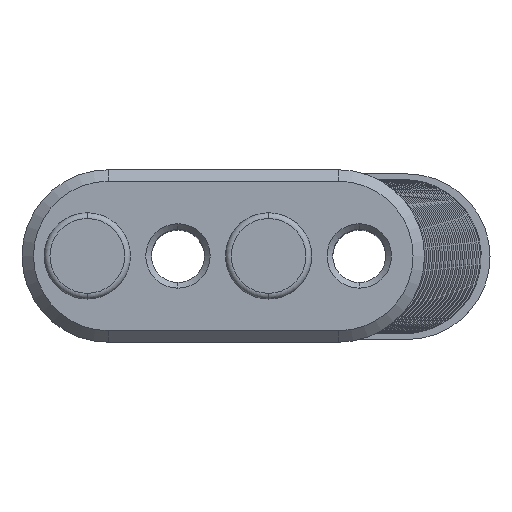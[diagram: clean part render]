
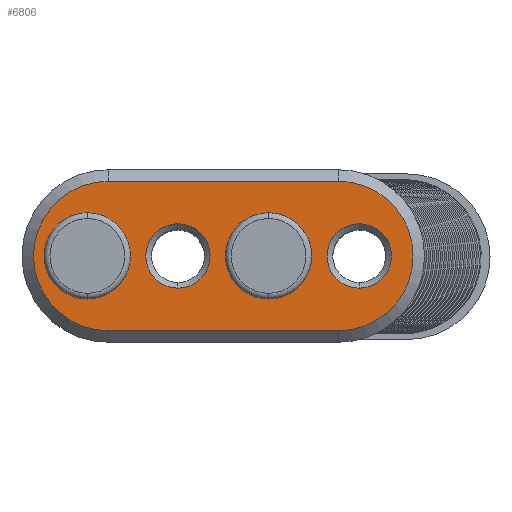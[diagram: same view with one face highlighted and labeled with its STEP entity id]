
A CAD part, top view. The second image highlights one B-rep face of the part: STEP entity #6806.
In plain terms, the highlighted planar face has unit normal (0, 0, 1).
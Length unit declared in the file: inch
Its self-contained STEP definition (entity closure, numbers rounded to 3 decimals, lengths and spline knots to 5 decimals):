
#20 = DIRECTION ( 'NONE',  ( 0., -1., 0. ) ) ;
#46 = EDGE_LOOP ( 'NONE', ( #3808, #5809 ) ) ;
#148 = FACE_BOUND ( 'NONE', #1703, .T. ) ;
#157 = AXIS2_PLACEMENT_3D ( 'NONE', #5842, #2017, #6483 ) ;
#225 = VERTEX_POINT ( 'NONE', #5051 ) ;
#270 = AXIS2_PLACEMENT_3D ( 'NONE', #5816, #649, #20 ) ;
#327 = DIRECTION ( 'NONE',  ( 0., 0., 1. ) ) ;
#331 = ORIENTED_EDGE ( 'NONE', *, *, #1484, .F. ) ;
#338 = DIRECTION ( 'NONE',  ( 0., 0., 1. ) ) ;
#632 = DIRECTION ( 'NONE',  ( 0., -1., 0. ) ) ;
#649 = DIRECTION ( 'NONE',  ( 0., 0., -1. ) ) ;
#738 = PLANE ( 'NONE',  #6042 ) ;
#747 = CARTESIAN_POINT ( 'NONE',  ( -0.5, -1.225, 1. ) ) ;
#770 = FACE_OUTER_BOUND ( 'NONE', #7071, .T. ) ;
#887 = VERTEX_POINT ( 'NONE', #1747 ) ;
#903 = DIRECTION ( 'NONE',  ( 0., 0., 1. ) ) ;
#988 = EDGE_CURVE ( 'NONE', #4217, #1450, #1202, .T. ) ;
#1107 = EDGE_CURVE ( 'NONE', #1518, #225, #6500, .T. ) ;
#1168 = AXIS2_PLACEMENT_3D ( 'NONE', #3433, #903, #4779 ) ;
#1202 = LINE ( 'NONE', #2324, #2707 ) ;
#1206 = EDGE_CURVE ( 'NONE', #1450, #887, #2096, .T. ) ;
#1263 = LINE ( 'NONE', #5788, #3372 ) ;
#1450 = VERTEX_POINT ( 'NONE', #3604 ) ;
#1484 = EDGE_CURVE ( 'NONE', #3655, #8273, #4808, .T. ) ;
#1518 = VERTEX_POINT ( 'NONE', #2064 ) ;
#1564 = VERTEX_POINT ( 'NONE', #6534 ) ;
#1665 = DIRECTION ( 'NONE',  ( 1., 0., 0. ) ) ;
#1668 = DIRECTION ( 'NONE',  ( 0., 0., 1. ) ) ;
#1703 = EDGE_LOOP ( 'NONE', ( #2561, #6641 ) ) ;
#1747 = CARTESIAN_POINT ( 'NONE',  ( 0.5, -0.575, 1. ) ) ;
#1845 = CIRCLE ( 'NONE', #2603, 0.14 ) ;
#1869 = FACE_BOUND ( 'NONE', #46, .T. ) ;
#1870 = CARTESIAN_POINT ( 'NONE',  ( -0.197, -0.9, 1. ) ) ;
#2017 = DIRECTION ( 'NONE',  ( 0., 0., 1. ) ) ;
#2064 = CARTESIAN_POINT ( 'NONE',  ( -0.197, -0.76, 1. ) ) ;
#2096 = CIRCLE ( 'NONE', #6592, 0.325 ) ;
#2220 = DIRECTION ( 'NONE',  ( 0., -1., 0. ) ) ;
#2307 = EDGE_CURVE ( 'NONE', #8273, #3655, #7782, .T. ) ;
#2324 = CARTESIAN_POINT ( 'NONE',  ( 0.5, -1.225, 1. ) ) ;
#2366 = CIRCLE ( 'NONE', #3315, 0.14 ) ;
#2367 = AXIS2_PLACEMENT_3D ( 'NONE', #8034, #1668, #6149 ) ;
#2561 = ORIENTED_EDGE ( 'NONE', *, *, #8281, .T. ) ;
#2574 = CARTESIAN_POINT ( 'NONE',  ( 0.197, -0.7125, 1. ) ) ;
#2603 = AXIS2_PLACEMENT_3D ( 'NONE', #1870, #6956, #632 ) ;
#2610 = ORIENTED_EDGE ( 'NONE', *, *, #5404, .T. ) ;
#2707 = VECTOR ( 'NONE', #1665, 39.37008 ) ;
#2919 = CARTESIAN_POINT ( 'NONE',  ( -0.5, -0.575, 1. ) ) ;
#3244 = ORIENTED_EDGE ( 'NONE', *, *, #6580, .T. ) ;
#3315 = AXIS2_PLACEMENT_3D ( 'NONE', #6217, #6987, #7657 ) ;
#3330 = CARTESIAN_POINT ( 'NONE',  ( -0.5, -0.9, 1. ) ) ;
#3372 = VECTOR ( 'NONE', #5237, 39.37008 ) ;
#3412 = AXIS2_PLACEMENT_3D ( 'NONE', #6832, #4358, #6253 ) ;
#3433 = CARTESIAN_POINT ( 'NONE',  ( -0.591, -0.9, 1. ) ) ;
#3521 = CARTESIAN_POINT ( 'NONE',  ( 0.5, -0.9, 1. ) ) ;
#3566 = EDGE_CURVE ( 'NONE', #7186, #1564, #5565, .T. ) ;
#3604 = CARTESIAN_POINT ( 'NONE',  ( 0.5, -1.225, 1. ) ) ;
#3655 = VERTEX_POINT ( 'NONE', #8133 ) ;
#3808 = ORIENTED_EDGE ( 'NONE', *, *, #3566, .F. ) ;
#3880 = ORIENTED_EDGE ( 'NONE', *, *, #5531, .T. ) ;
#3894 = DIRECTION ( 'NONE',  ( 0., -1., 0. ) ) ;
#4038 = DIRECTION ( 'NONE',  ( 0., -1., 0. ) ) ;
#4188 = FACE_BOUND ( 'NONE', #4301, .T. ) ;
#4217 = VERTEX_POINT ( 'NONE', #747 ) ;
#4301 = EDGE_LOOP ( 'NONE', ( #3244, #3880 ) ) ;
#4358 = DIRECTION ( 'NONE',  ( 0., 0., 1. ) ) ;
#4389 = CARTESIAN_POINT ( 'NONE',  ( -0.591, -0.7125, 1. ) ) ;
#4605 = EDGE_CURVE ( 'NONE', #887, #7717, #1263, .T. ) ;
#4779 = DIRECTION ( 'NONE',  ( 0., -1., 0. ) ) ;
#4808 = CIRCLE ( 'NONE', #2367, 0.1875 ) ;
#5051 = CARTESIAN_POINT ( 'NONE',  ( -0.197, -1.04, 1. ) ) ;
#5233 = CARTESIAN_POINT ( 'NONE',  ( 0.591, -0.76, 1. ) ) ;
#5237 = DIRECTION ( 'NONE',  ( -1., 0., 0. ) ) ;
#5239 = DIRECTION ( 'NONE',  ( 0., 0., 1. ) ) ;
#5247 = EDGE_CURVE ( 'NONE', #1564, #7186, #6453, .T. ) ;
#5267 = CARTESIAN_POINT ( 'NONE',  ( -0.197, -0.9, 1. ) ) ;
#5404 = EDGE_CURVE ( 'NONE', #7717, #4217, #6057, .T. ) ;
#5524 = ORIENTED_EDGE ( 'NONE', *, *, #4605, .T. ) ;
#5531 = EDGE_CURVE ( 'NONE', #7368, #5681, #5954, .T. ) ;
#5565 = CIRCLE ( 'NONE', #1168, 0.1875 ) ;
#5681 = VERTEX_POINT ( 'NONE', #7916 ) ;
#5788 = CARTESIAN_POINT ( 'NONE',  ( -0.5, -0.575, 1. ) ) ;
#5809 = ORIENTED_EDGE ( 'NONE', *, *, #5247, .F. ) ;
#5816 = CARTESIAN_POINT ( 'NONE',  ( 0.591, -0.9, 1. ) ) ;
#5842 = CARTESIAN_POINT ( 'NONE',  ( 0.197, -0.9, 1. ) ) ;
#5954 = CIRCLE ( 'NONE', #270, 0.14 ) ;
#6027 = AXIS2_PLACEMENT_3D ( 'NONE', #5267, #6030, #4038 ) ;
#6030 = DIRECTION ( 'NONE',  ( 0., 0., -1. ) ) ;
#6042 = AXIS2_PLACEMENT_3D ( 'NONE', #3330, #5239, #3894 ) ;
#6057 = CIRCLE ( 'NONE', #3412, 0.325 ) ;
#6129 = DIRECTION ( 'NONE',  ( 0., -1., 0. ) ) ;
#6149 = DIRECTION ( 'NONE',  ( 0., -1., 0. ) ) ;
#6217 = CARTESIAN_POINT ( 'NONE',  ( 0.591, -0.9, 1. ) ) ;
#6253 = DIRECTION ( 'NONE',  ( 0., -1., 0. ) ) ;
#6318 = ORIENTED_EDGE ( 'NONE', *, *, #2307, .F. ) ;
#6385 = ORIENTED_EDGE ( 'NONE', *, *, #1206, .T. ) ;
#6453 = CIRCLE ( 'NONE', #7831, 0.1875 ) ;
#6483 = DIRECTION ( 'NONE',  ( 0., -1., 0. ) ) ;
#6500 = CIRCLE ( 'NONE', #6027, 0.14 ) ;
#6534 = CARTESIAN_POINT ( 'NONE',  ( -0.591, -1.0875, 1. ) ) ;
#6580 = EDGE_CURVE ( 'NONE', #5681, #7368, #2366, .T. ) ;
#6592 = AXIS2_PLACEMENT_3D ( 'NONE', #3521, #338, #2220 ) ;
#6641 = ORIENTED_EDGE ( 'NONE', *, *, #1107, .T. ) ;
#6763 = FACE_BOUND ( 'NONE', #6866, .T. ) ;
#6806 = ADVANCED_FACE ( 'NONE', ( #148, #4188, #770, #1869, #6763 ), #738, .T. ) ;
#6832 = CARTESIAN_POINT ( 'NONE',  ( -0.5, -0.9, 1. ) ) ;
#6866 = EDGE_LOOP ( 'NONE', ( #6318, #331 ) ) ;
#6956 = DIRECTION ( 'NONE',  ( 0., 0., -1. ) ) ;
#6987 = DIRECTION ( 'NONE',  ( 0., 0., -1. ) ) ;
#7071 = EDGE_LOOP ( 'NONE', ( #6385, #5524, #2610, #7889 ) ) ;
#7186 = VERTEX_POINT ( 'NONE', #4389 ) ;
#7368 = VERTEX_POINT ( 'NONE', #5233 ) ;
#7657 = DIRECTION ( 'NONE',  ( 0., -1., 0. ) ) ;
#7717 = VERTEX_POINT ( 'NONE', #2919 ) ;
#7782 = CIRCLE ( 'NONE', #157, 0.1875 ) ;
#7831 = AXIS2_PLACEMENT_3D ( 'NONE', #8095, #327, #6129 ) ;
#7889 = ORIENTED_EDGE ( 'NONE', *, *, #988, .T. ) ;
#7916 = CARTESIAN_POINT ( 'NONE',  ( 0.591, -1.04, 1. ) ) ;
#8034 = CARTESIAN_POINT ( 'NONE',  ( 0.197, -0.9, 1. ) ) ;
#8095 = CARTESIAN_POINT ( 'NONE',  ( -0.591, -0.9, 1. ) ) ;
#8133 = CARTESIAN_POINT ( 'NONE',  ( 0.197, -1.0875, 1. ) ) ;
#8273 = VERTEX_POINT ( 'NONE', #2574 ) ;
#8281 = EDGE_CURVE ( 'NONE', #225, #1518, #1845, .T. ) ;
